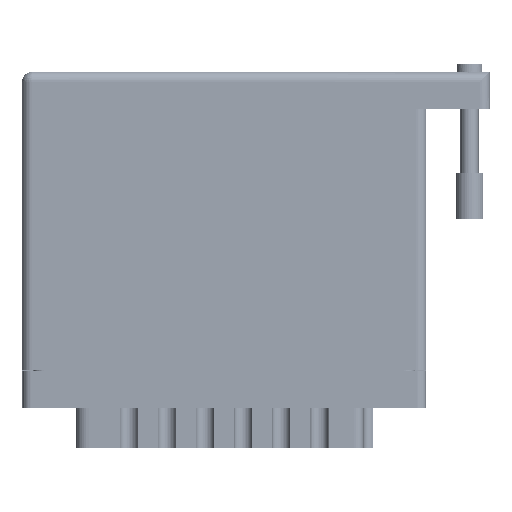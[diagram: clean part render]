
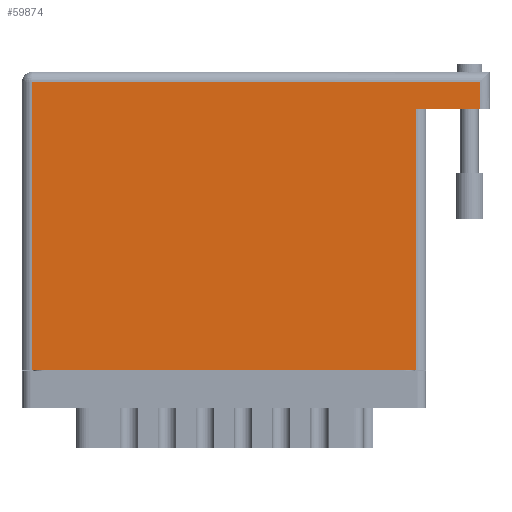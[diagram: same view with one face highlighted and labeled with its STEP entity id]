
A CAD part, front view. The second image highlights one B-rep face of the part: STEP entity #59874.
In plain terms, the highlighted face is planar.
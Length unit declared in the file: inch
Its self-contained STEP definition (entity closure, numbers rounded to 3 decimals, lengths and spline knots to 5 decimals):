
#911 = VECTOR ( 'NONE', #38844, 39.37008 ) ;
#3402 = VERTEX_POINT ( 'NONE', #54024 ) ;
#3556 = VERTEX_POINT ( 'NONE', #56782 ) ;
#4446 = VERTEX_POINT ( 'NONE', #6196 ) ;
#4679 = CARTESIAN_POINT ( 'NONE',  ( 0.07, 1.96, 0. ) ) ;
#5551 = LINE ( 'NONE', #88318, #81748 ) ;
#6196 = CARTESIAN_POINT ( 'NONE',  ( 2.685, 1.774, 0. ) ) ;
#10079 = CARTESIAN_POINT ( 'NONE',  ( 0., 0., 0. ) ) ;
#12499 = FACE_OUTER_BOUND ( 'NONE', #92235, .T. ) ;
#14078 = ORIENTED_EDGE ( 'NONE', *, *, #55371, .T. ) ;
#16727 = LINE ( 'NONE', #77484, #82853 ) ;
#18814 = DIRECTION ( 'NONE',  ( -1., 0., 0. ) ) ;
#19411 = DIRECTION ( 'NONE',  ( 0., 1., 0. ) ) ;
#21958 = VECTOR ( 'NONE', #47053, 39.37008 ) ;
#23339 = VERTEX_POINT ( 'NONE', #32288 ) ;
#24171 = CARTESIAN_POINT ( 'NONE',  ( 0.07, 0., 0. ) ) ;
#27760 = ORIENTED_EDGE ( 'NONE', *, *, #75554, .T. ) ;
#30896 = LINE ( 'NONE', #10079, #21958 ) ;
#32288 = CARTESIAN_POINT ( 'NONE',  ( 2.685, 0., 0. ) ) ;
#33199 = DIRECTION ( 'NONE',  ( -1., 0., 0. ) ) ;
#36036 = ORIENTED_EDGE ( 'NONE', *, *, #77317, .T. ) ;
#37496 = LINE ( 'NONE', #54545, #73399 ) ;
#38844 = DIRECTION ( 'NONE',  ( 0., -1., 0. ) ) ;
#45065 = CARTESIAN_POINT ( 'NONE',  ( 3.12, 1.774, 0. ) ) ;
#47053 = DIRECTION ( 'NONE',  ( 1., 0., 0. ) ) ;
#47402 = VERTEX_POINT ( 'NONE', #4679 ) ;
#48950 = EDGE_CURVE ( 'NONE', #47402, #3402, #60460, .T. ) ;
#51561 = LINE ( 'NONE', #76422, #90675 ) ;
#54024 = CARTESIAN_POINT ( 'NONE',  ( 0.07, 0., 0. ) ) ;
#54545 = CARTESIAN_POINT ( 'NONE',  ( 0., 1.96, 0. ) ) ;
#55371 = EDGE_CURVE ( 'NONE', #23339, #4446, #51561, .T. ) ;
#56782 = CARTESIAN_POINT ( 'NONE',  ( 3.12, 1.96, 0. ) ) ;
#59874 = ADVANCED_FACE ( 'NONE', ( #12499 ), #92003, .F. ) ;
#60460 = LINE ( 'NONE', #24171, #911 ) ;
#60721 = AXIS2_PLACEMENT_3D ( 'NONE', #71704, #79141, #78846 ) ;
#63754 = DIRECTION ( 'NONE',  ( 0., 1., 0. ) ) ;
#70276 = ORIENTED_EDGE ( 'NONE', *, *, #91773, .F. ) ;
#71704 = CARTESIAN_POINT ( 'NONE',  ( 0., 2.03, 0. ) ) ;
#73399 = VECTOR ( 'NONE', #33199, 39.37008 ) ;
#75554 = EDGE_CURVE ( 'NONE', #3556, #47402, #37496, .T. ) ;
#76422 = CARTESIAN_POINT ( 'NONE',  ( 2.685, 1.774, 0. ) ) ;
#77317 = EDGE_CURVE ( 'NONE', #3402, #23339, #30896, .T. ) ;
#77484 = CARTESIAN_POINT ( 'NONE',  ( 3.12, 2.03, 0. ) ) ;
#77627 = ORIENTED_EDGE ( 'NONE', *, *, #48950, .T. ) ;
#78846 = DIRECTION ( 'NONE',  ( -1., 0., 0. ) ) ;
#79141 = DIRECTION ( 'NONE',  ( 0., 0., -1. ) ) ;
#80605 = EDGE_CURVE ( 'NONE', #92374, #3556, #16727, .T. ) ;
#81748 = VECTOR ( 'NONE', #18814, 39.37008 ) ;
#82853 = VECTOR ( 'NONE', #63754, 39.37008 ) ;
#84895 = ORIENTED_EDGE ( 'NONE', *, *, #80605, .T. ) ;
#88318 = CARTESIAN_POINT ( 'NONE',  ( 3.19, 1.774, 0. ) ) ;
#90675 = VECTOR ( 'NONE', #19411, 39.37008 ) ;
#91773 = EDGE_CURVE ( 'NONE', #92374, #4446, #5551, .T. ) ;
#92003 = PLANE ( 'NONE',  #60721 ) ;
#92235 = EDGE_LOOP ( 'NONE', ( #36036, #14078, #70276, #84895, #27760, #77627 ) ) ;
#92374 = VERTEX_POINT ( 'NONE', #45065 ) ;
